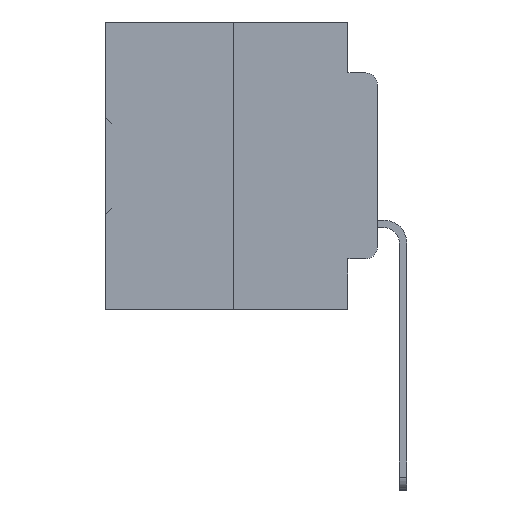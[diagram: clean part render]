
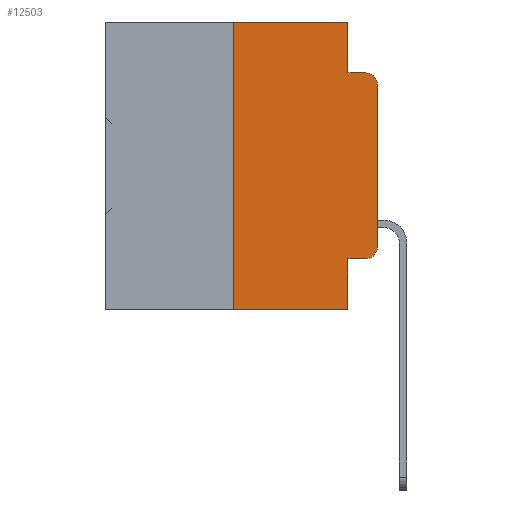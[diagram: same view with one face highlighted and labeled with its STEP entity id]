
A CAD part, left-side view. The second image highlights one B-rep face of the part: STEP entity #12503.
In plain terms, the highlighted planar face has unit normal (-1, 0, 0).
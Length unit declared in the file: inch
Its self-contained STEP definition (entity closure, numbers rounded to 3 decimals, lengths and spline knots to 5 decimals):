
#519 = VECTOR ( 'NONE', #3397, 39.37008 ) ;
#744 = DIRECTION ( 'NONE',  ( 0., 0., -1. ) ) ;
#1087 = CARTESIAN_POINT ( 'NONE',  ( 0., 0., 0. ) ) ;
#1303 = EDGE_CURVE ( 'NONE', #38069, #32929, #10887, .T. ) ;
#2531 = CARTESIAN_POINT ( 'NONE',  ( 0., 0.02, -0.3915 ) ) ;
#2817 = LINE ( 'NONE', #27293, #9967 ) ;
#3397 = DIRECTION ( 'NONE',  ( 0., -1., 0. ) ) ;
#4741 = VERTEX_POINT ( 'NONE', #14430 ) ;
#5236 = CARTESIAN_POINT ( 'NONE',  ( 0., 0.473, 0. ) ) ;
#5626 = DIRECTION ( 'NONE',  ( 0., 0., -1. ) ) ;
#7222 = LINE ( 'NONE', #1087, #30835 ) ;
#7287 = CARTESIAN_POINT ( 'NONE',  ( 0., 0.25, -0.5 ) ) ;
#8111 = FACE_OUTER_BOUND ( 'NONE', #11031, .T. ) ;
#8198 = CARTESIAN_POINT ( 'NONE',  ( 0., 0.051, 0. ) ) ;
#8315 = DIRECTION ( 'NONE',  ( 0., 0., -1. ) ) ;
#9039 = VERTEX_POINT ( 'NONE', #34385 ) ;
#9348 = CARTESIAN_POINT ( 'NONE',  ( 0., 0.02, -0.4115 ) ) ;
#9967 = VECTOR ( 'NONE', #24385, 39.37008 ) ;
#10733 = VERTEX_POINT ( 'NONE', #7287 ) ;
#10788 = CARTESIAN_POINT ( 'NONE',  ( 0., 0.051, 0. ) ) ;
#10805 = ORIENTED_EDGE ( 'NONE', *, *, #30079, .F. ) ;
#10887 = LINE ( 'NONE', #8198, #34326 ) ;
#10928 = AXIS2_PLACEMENT_3D ( 'NONE', #5236, #26090, #8315 ) ;
#11031 = EDGE_LOOP ( 'NONE', ( #37874, #17359, #25131, #21013, #36500, #38349, #31526, #10805, #34247, #27008 ) ) ;
#11060 = DIRECTION ( 'NONE',  ( 0., -1., 0. ) ) ;
#12503 = ADVANCED_FACE ( 'NONE', ( #8111 ), #34736, .F. ) ;
#12589 = VERTEX_POINT ( 'NONE', #23410 ) ;
#12906 = VERTEX_POINT ( 'NONE', #18887 ) ;
#13847 = DIRECTION ( 'NONE',  ( 0., 0., -1. ) ) ;
#14106 = CARTESIAN_POINT ( 'NONE',  ( 0., 0.473, 0. ) ) ;
#14232 = DIRECTION ( 'NONE',  ( -1., 0., 0. ) ) ;
#14430 = CARTESIAN_POINT ( 'NONE',  ( 0., 0., -0.3915 ) ) ;
#14896 = EDGE_CURVE ( 'NONE', #12589, #21812, #33740, .T. ) ;
#15784 = DIRECTION ( 'NONE',  ( 0., -1., 0. ) ) ;
#16883 = EDGE_CURVE ( 'NONE', #4741, #12589, #7222, .T. ) ;
#17359 = ORIENTED_EDGE ( 'NONE', *, *, #14896, .T. ) ;
#18213 = VERTEX_POINT ( 'NONE', #37379 ) ;
#18334 = EDGE_CURVE ( 'NONE', #18489, #4741, #30260, .T. ) ;
#18489 = VERTEX_POINT ( 'NONE', #9348 ) ;
#18610 = EDGE_CURVE ( 'NONE', #10733, #12906, #21996, .T. ) ;
#18756 = CARTESIAN_POINT ( 'NONE',  ( 0., 0.473, -0.5 ) ) ;
#18887 = CARTESIAN_POINT ( 'NONE',  ( 0., 0.051, -0.5 ) ) ;
#20794 = VECTOR ( 'NONE', #13847, 39.37008 ) ;
#21013 = ORIENTED_EDGE ( 'NONE', *, *, #1303, .F. ) ;
#21103 = VECTOR ( 'NONE', #15784, 39.37008 ) ;
#21812 = VERTEX_POINT ( 'NONE', #24655 ) ;
#21996 = LINE ( 'NONE', #18756, #21103 ) ;
#22066 = EDGE_CURVE ( 'NONE', #9039, #38069, #32105, .T. ) ;
#22183 = DIRECTION ( 'NONE',  ( 0., 0., 1. ) ) ;
#22231 = EDGE_CURVE ( 'NONE', #18213, #18489, #33439, .T. ) ;
#23410 = CARTESIAN_POINT ( 'NONE',  ( 0., 0., -0.1085 ) ) ;
#23520 = CARTESIAN_POINT ( 'NONE',  ( 0., 0.051, 0. ) ) ;
#23540 = DIRECTION ( 'NONE',  ( -1., 0., 0. ) ) ;
#24385 = DIRECTION ( 'NONE',  ( 0., 0., 1. ) ) ;
#24655 = CARTESIAN_POINT ( 'NONE',  ( 0., 0.02, -0.0885 ) ) ;
#25131 = ORIENTED_EDGE ( 'NONE', *, *, #25460, .F. ) ;
#25460 = EDGE_CURVE ( 'NONE', #32929, #21812, #32336, .T. ) ;
#26090 = DIRECTION ( 'NONE',  ( 1., 0., 0. ) ) ;
#27008 = ORIENTED_EDGE ( 'NONE', *, *, #18334, .T. ) ;
#27293 = CARTESIAN_POINT ( 'NONE',  ( 0., 0.25, 0. ) ) ;
#28566 = LINE ( 'NONE', #10788, #20794 ) ;
#30079 = EDGE_CURVE ( 'NONE', #18213, #12906, #28566, .T. ) ;
#30260 = CIRCLE ( 'NONE', #36374, 0.02 ) ;
#30835 = VECTOR ( 'NONE', #22183, 39.37008 ) ;
#31172 = VECTOR ( 'NONE', #11060, 39.37008 ) ;
#31526 = ORIENTED_EDGE ( 'NONE', *, *, #18610, .T. ) ;
#31759 = CARTESIAN_POINT ( 'NONE',  ( 0., 0.02, -0.1085 ) ) ;
#32042 = EDGE_CURVE ( 'NONE', #10733, #9039, #2817, .T. ) ;
#32105 = LINE ( 'NONE', #14106, #31172 ) ;
#32336 = LINE ( 'NONE', #32987, #519 ) ;
#32929 = VERTEX_POINT ( 'NONE', #34337 ) ;
#32987 = CARTESIAN_POINT ( 'NONE',  ( 0., 0.051, -0.0885 ) ) ;
#33439 = LINE ( 'NONE', #38373, #34345 ) ;
#33740 = CIRCLE ( 'NONE', #35355, 0.02 ) ;
#34247 = ORIENTED_EDGE ( 'NONE', *, *, #22231, .T. ) ;
#34326 = VECTOR ( 'NONE', #744, 39.37008 ) ;
#34337 = CARTESIAN_POINT ( 'NONE',  ( 0., 0.051, -0.0885 ) ) ;
#34345 = VECTOR ( 'NONE', #38245, 39.37008 ) ;
#34385 = CARTESIAN_POINT ( 'NONE',  ( 0., 0.25, 0. ) ) ;
#34691 = DIRECTION ( 'NONE',  ( 0., 0., -1. ) ) ;
#34736 = PLANE ( 'NONE',  #10928 ) ;
#35355 = AXIS2_PLACEMENT_3D ( 'NONE', #31759, #14232, #34691 ) ;
#36374 = AXIS2_PLACEMENT_3D ( 'NONE', #2531, #23540, #5626 ) ;
#36500 = ORIENTED_EDGE ( 'NONE', *, *, #22066, .F. ) ;
#37379 = CARTESIAN_POINT ( 'NONE',  ( 0., 0.051, -0.4115 ) ) ;
#37874 = ORIENTED_EDGE ( 'NONE', *, *, #16883, .T. ) ;
#38069 = VERTEX_POINT ( 'NONE', #23520 ) ;
#38245 = DIRECTION ( 'NONE',  ( 0., -1., 0. ) ) ;
#38349 = ORIENTED_EDGE ( 'NONE', *, *, #32042, .F. ) ;
#38373 = CARTESIAN_POINT ( 'NONE',  ( 0., 0.051, -0.4115 ) ) ;
